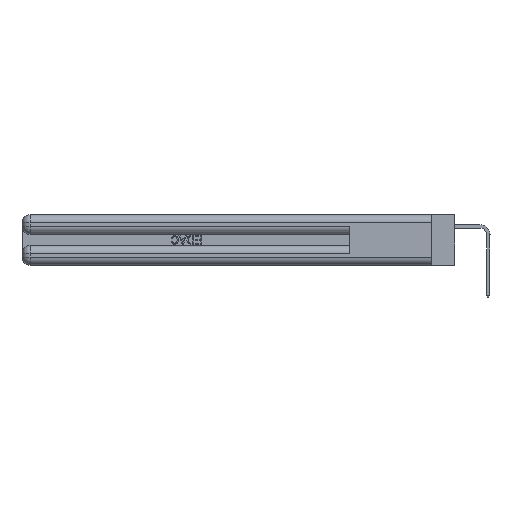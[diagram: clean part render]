
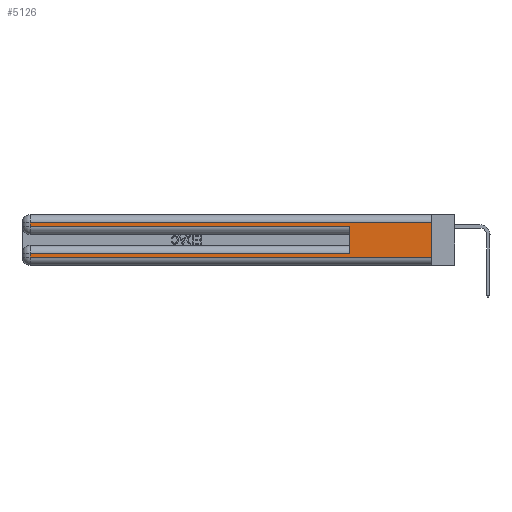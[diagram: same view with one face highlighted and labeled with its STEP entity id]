
A CAD part, left-side view. The second image highlights one B-rep face of the part: STEP entity #5126.
In plain terms, the highlighted planar face has unit normal (-1, 0, 0).
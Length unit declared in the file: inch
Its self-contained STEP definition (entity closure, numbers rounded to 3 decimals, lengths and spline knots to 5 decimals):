
#1193 = VERTEX_POINT ( 'NONE', #9161 ) ;
#1882 = FACE_OUTER_BOUND ( 'NONE', #7514, .T. ) ;
#2167 = EDGE_CURVE ( 'NONE', #1193, #5858, #5748, .T. ) ;
#2974 = ORIENTED_EDGE ( 'NONE', *, *, #29079, .T. ) ;
#3093 = EDGE_CURVE ( 'NONE', #17205, #5858, #25789, .T. ) ;
#3503 = VECTOR ( 'NONE', #38837, 39.37008 ) ;
#5126 = ADVANCED_FACE ( 'NONE', ( #1882 ), #39221, .F. ) ;
#5748 = LINE ( 'NONE', #19426, #45813 ) ;
#5858 = VERTEX_POINT ( 'NONE', #24342 ) ;
#6616 = LINE ( 'NONE', #11275, #46671 ) ;
#7427 = EDGE_CURVE ( 'NONE', #33878, #45849, #47276, .T. ) ;
#7514 = EDGE_LOOP ( 'NONE', ( #33218, #20876, #2974, #34411, #29826, #14470, #48752, #37208 ) ) ;
#7518 = DIRECTION ( 'NONE',  ( 0., 0., 1. ) ) ;
#7528 = CARTESIAN_POINT ( 'NONE',  ( 0., 0., 0.31 ) ) ;
#7529 = CARTESIAN_POINT ( 'NONE',  ( 0., 0., 0.085 ) ) ;
#9161 = CARTESIAN_POINT ( 'NONE',  ( 0., 0.6, 0.085 ) ) ;
#9775 = EDGE_CURVE ( 'NONE', #42541, #11356, #15460, .T. ) ;
#10402 = CARTESIAN_POINT ( 'NONE',  ( 0., 2.94, 0.285 ) ) ;
#11275 = CARTESIAN_POINT ( 'NONE',  ( 0., 0., 0.37 ) ) ;
#11356 = VERTEX_POINT ( 'NONE', #42144 ) ;
#11482 = DIRECTION ( 'NONE',  ( 0., 0., -1. ) ) ;
#13622 = VECTOR ( 'NONE', #30237, 39.37008 ) ;
#13906 = VECTOR ( 'NONE', #33115, 39.37008 ) ;
#14470 = ORIENTED_EDGE ( 'NONE', *, *, #18313, .T. ) ;
#14954 = CARTESIAN_POINT ( 'NONE',  ( 0., 0., 0.06 ) ) ;
#15460 = LINE ( 'NONE', #7528, #44834 ) ;
#17205 = VERTEX_POINT ( 'NONE', #10402 ) ;
#18313 = EDGE_CURVE ( 'NONE', #1193, #39136, #36485, .T. ) ;
#18890 = LINE ( 'NONE', #33459, #49542 ) ;
#19426 = CARTESIAN_POINT ( 'NONE',  ( 0., 0.6, 0.145 ) ) ;
#20540 = CARTESIAN_POINT ( 'NONE',  ( 0., 2.94, 0.085 ) ) ;
#20876 = ORIENTED_EDGE ( 'NONE', *, *, #9775, .T. ) ;
#21085 = CARTESIAN_POINT ( 'NONE',  ( 0., 0., 0.285 ) ) ;
#23113 = CARTESIAN_POINT ( 'NONE',  ( 0., 2.94, 0.06 ) ) ;
#23373 = CARTESIAN_POINT ( 'NONE',  ( 0., 0., 0.37 ) ) ;
#24243 = LINE ( 'NONE', #50181, #13622 ) ;
#24342 = CARTESIAN_POINT ( 'NONE',  ( 0., 0.6, 0.285 ) ) ;
#24434 = EDGE_CURVE ( 'NONE', #39136, #33878, #18890, .T. ) ;
#25789 = LINE ( 'NONE', #21085, #13906 ) ;
#27081 = VECTOR ( 'NONE', #35474, 39.37008 ) ;
#27826 = CARTESIAN_POINT ( 'NONE',  ( 0., 0., 0.31 ) ) ;
#29079 = EDGE_CURVE ( 'NONE', #11356, #17205, #24243, .T. ) ;
#29826 = ORIENTED_EDGE ( 'NONE', *, *, #2167, .F. ) ;
#30237 = DIRECTION ( 'NONE',  ( 0., 0., -1. ) ) ;
#31465 = DIRECTION ( 'NONE',  ( 0., 1., 0. ) ) ;
#33115 = DIRECTION ( 'NONE',  ( 0., -1., 0. ) ) ;
#33218 = ORIENTED_EDGE ( 'NONE', *, *, #35093, .F. ) ;
#33459 = CARTESIAN_POINT ( 'NONE',  ( 0., 2.94, 0.37 ) ) ;
#33878 = VERTEX_POINT ( 'NONE', #23113 ) ;
#34411 = ORIENTED_EDGE ( 'NONE', *, *, #3093, .T. ) ;
#35093 = EDGE_CURVE ( 'NONE', #42541, #45849, #6616, .T. ) ;
#35407 = DIRECTION ( 'NONE',  ( 1., 0., 0. ) ) ;
#35474 = DIRECTION ( 'NONE',  ( 0., 1., 0. ) ) ;
#36485 = LINE ( 'NONE', #7529, #27081 ) ;
#37208 = ORIENTED_EDGE ( 'NONE', *, *, #7427, .T. ) ;
#38837 = DIRECTION ( 'NONE',  ( 0., -1., 0. ) ) ;
#39136 = VERTEX_POINT ( 'NONE', #20540 ) ;
#39221 = PLANE ( 'NONE',  #50183 ) ;
#39372 = DIRECTION ( 'NONE',  ( 0., 0., -1. ) ) ;
#42144 = CARTESIAN_POINT ( 'NONE',  ( 0., 2.94, 0.31 ) ) ;
#42541 = VERTEX_POINT ( 'NONE', #27826 ) ;
#44834 = VECTOR ( 'NONE', #31465, 39.37008 ) ;
#45371 = DIRECTION ( 'NONE',  ( 0., 0., -1. ) ) ;
#45813 = VECTOR ( 'NONE', #7518, 39.37008 ) ;
#45849 = VERTEX_POINT ( 'NONE', #49724 ) ;
#46671 = VECTOR ( 'NONE', #39372, 39.37008 ) ;
#47276 = LINE ( 'NONE', #14954, #3503 ) ;
#48752 = ORIENTED_EDGE ( 'NONE', *, *, #24434, .T. ) ;
#49542 = VECTOR ( 'NONE', #45371, 39.37008 ) ;
#49724 = CARTESIAN_POINT ( 'NONE',  ( 0., 0., 0.06 ) ) ;
#50181 = CARTESIAN_POINT ( 'NONE',  ( 0., 2.94, 0.37 ) ) ;
#50183 = AXIS2_PLACEMENT_3D ( 'NONE', #23373, #35407, #11482 ) ;
